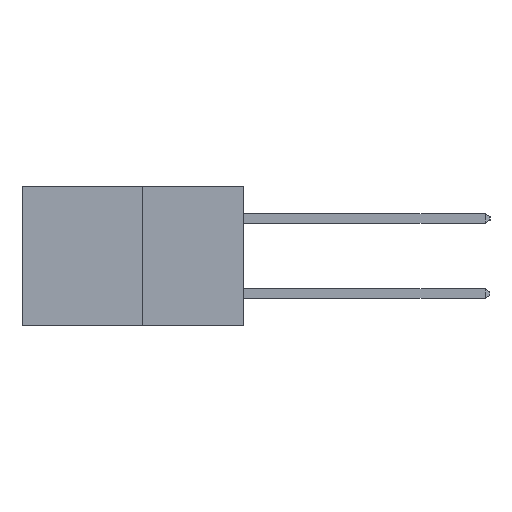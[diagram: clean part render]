
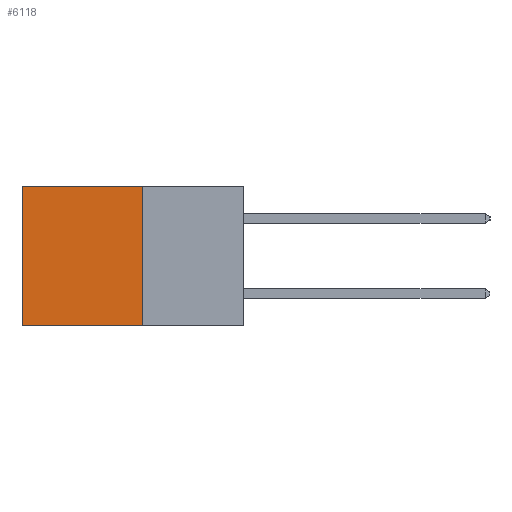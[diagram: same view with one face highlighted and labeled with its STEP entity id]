
A CAD part, left-side view. The second image highlights one B-rep face of the part: STEP entity #6118.
In plain terms, the highlighted planar face has unit normal (-1, 0, 0).
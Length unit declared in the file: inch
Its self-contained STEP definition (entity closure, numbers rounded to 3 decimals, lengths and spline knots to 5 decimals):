
#2 = ORIENTED_EDGE ( 'NONE', *, *, #11768, .F. ) ;
#430 = ORIENTED_EDGE ( 'NONE', *, *, #6167, .F. ) ;
#481 = ORIENTED_EDGE ( 'NONE', *, *, #8887, .T. ) ;
#936 = EDGE_CURVE ( 'NONE', #5628, #4212, #4465, .T. ) ;
#1458 = VECTOR ( 'NONE', #10056, 39.37008 ) ;
#2036 = VECTOR ( 'NONE', #12105, 39.37008 ) ;
#2419 = LINE ( 'NONE', #11088, #2036 ) ;
#3030 = EDGE_LOOP ( 'NONE', ( #11476, #2, #430, #481 ) ) ;
#3372 = CARTESIAN_POINT ( 'NONE',  ( 0.277, 0.59, -0.37 ) ) ;
#3529 = DIRECTION ( 'NONE',  ( 0., 1., 0. ) ) ;
#4212 = VERTEX_POINT ( 'NONE', #5711 ) ;
#4465 = LINE ( 'NONE', #3372, #1458 ) ;
#4745 = CARTESIAN_POINT ( 'NONE',  ( 0.277, 0.27, -0.37 ) ) ;
#5628 = VERTEX_POINT ( 'NONE', #7160 ) ;
#5702 = PLANE ( 'NONE',  #11095 ) ;
#5711 = CARTESIAN_POINT ( 'NONE',  ( 0.277, 0.59, -0.37 ) ) ;
#5786 = VECTOR ( 'NONE', #11884, 39.37008 ) ;
#6118 = ADVANCED_FACE ( 'NONE', ( #8481 ), #5702, .F. ) ;
#6167 = EDGE_CURVE ( 'NONE', #12670, #7630, #13578, .T. ) ;
#6598 = VECTOR ( 'NONE', #3529, 39.37008 ) ;
#6732 = DIRECTION ( 'NONE',  ( 0., 0., -1. ) ) ;
#6900 = LINE ( 'NONE', #11723, #6598 ) ;
#7160 = CARTESIAN_POINT ( 'NONE',  ( 0.277, 0.59, 0. ) ) ;
#7630 = VERTEX_POINT ( 'NONE', #13461 ) ;
#8481 = FACE_OUTER_BOUND ( 'NONE', #3030, .T. ) ;
#8887 = EDGE_CURVE ( 'NONE', #12670, #5628, #2419, .T. ) ;
#9694 = CARTESIAN_POINT ( 'NONE',  ( 0.277, 0.27, 0. ) ) ;
#9782 = CARTESIAN_POINT ( 'NONE',  ( 0.277, 0.27, -0.37 ) ) ;
#10056 = DIRECTION ( 'NONE',  ( 0., 0., -1. ) ) ;
#11088 = CARTESIAN_POINT ( 'NONE',  ( 0.277, 0.27, 0. ) ) ;
#11095 = AXIS2_PLACEMENT_3D ( 'NONE', #9782, #12869, #6732 ) ;
#11476 = ORIENTED_EDGE ( 'NONE', *, *, #936, .T. ) ;
#11723 = CARTESIAN_POINT ( 'NONE',  ( 0.277, 0.27, -0.37 ) ) ;
#11768 = EDGE_CURVE ( 'NONE', #7630, #4212, #6900, .T. ) ;
#11884 = DIRECTION ( 'NONE',  ( 0., 0., -1. ) ) ;
#12105 = DIRECTION ( 'NONE',  ( 0., 1., 0. ) ) ;
#12670 = VERTEX_POINT ( 'NONE', #9694 ) ;
#12869 = DIRECTION ( 'NONE',  ( 1., 0., 0. ) ) ;
#13461 = CARTESIAN_POINT ( 'NONE',  ( 0.277, 0.27, -0.37 ) ) ;
#13578 = LINE ( 'NONE', #4745, #5786 ) ;
